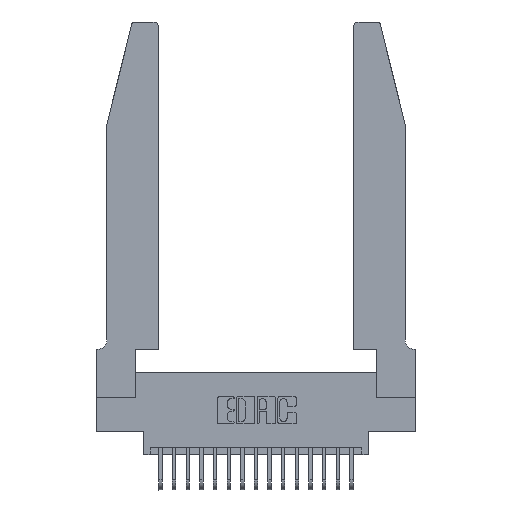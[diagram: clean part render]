
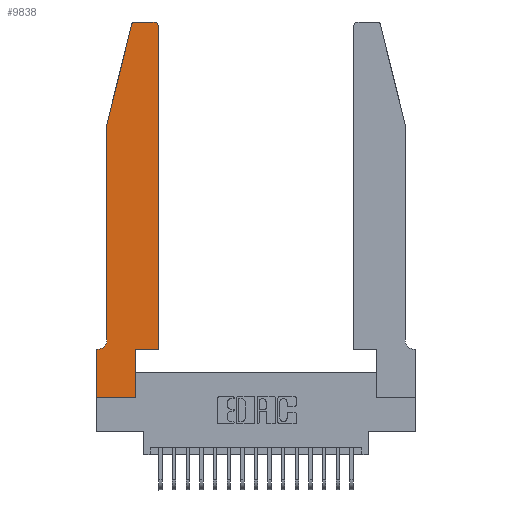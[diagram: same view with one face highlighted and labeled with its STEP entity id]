
A CAD part, top view. The second image highlights one B-rep face of the part: STEP entity #9838.
In plain terms, the highlighted planar face has unit normal (0, 0, 1).
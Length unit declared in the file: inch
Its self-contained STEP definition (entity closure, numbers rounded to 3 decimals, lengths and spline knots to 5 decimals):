
#3 = VERTEX_POINT ( 'NONE', #16463 ) ;
#255 = EDGE_CURVE ( 'NONE', #14930, #7111, #9008, .T. ) ;
#265 = CARTESIAN_POINT ( 'NONE',  ( 0.284, 2.75, 0.37 ) ) ;
#347 = CARTESIAN_POINT ( 'NONE',  ( 0.284, 2.72, 0.37 ) ) ;
#1038 = DIRECTION ( 'NONE',  ( 0., 0., 1. ) ) ;
#1170 = ORIENTED_EDGE ( 'NONE', *, *, #16123, .T. ) ;
#1214 = DIRECTION ( 'NONE',  ( 0., 1., 0. ) ) ;
#1330 = VECTOR ( 'NONE', #4417, 39.37008 ) ;
#1335 = DIRECTION ( 'NONE',  ( 1., 0., 0. ) ) ;
#1813 = VERTEX_POINT ( 'NONE', #8949 ) ;
#1991 = ORIENTED_EDGE ( 'NONE', *, *, #9637, .T. ) ;
#2097 = CARTESIAN_POINT ( 'NONE',  ( 0.4505, 2.72, 0.37 ) ) ;
#2104 = ORIENTED_EDGE ( 'NONE', *, *, #6098, .T. ) ;
#2173 = VECTOR ( 'NONE', #8226, 39.37008 ) ;
#2244 = EDGE_CURVE ( 'NONE', #2578, #7354, #13419, .T. ) ;
#2578 = VERTEX_POINT ( 'NONE', #265 ) ;
#2628 = EDGE_CURVE ( 'NONE', #7111, #5999, #11754, .T. ) ;
#2668 = LINE ( 'NONE', #11325, #2173 ) ;
#2983 = VECTOR ( 'NONE', #9840, 39.37008 ) ;
#3103 = AXIS2_PLACEMENT_3D ( 'NONE', #19707, #10705, #1335 ) ;
#3227 = CARTESIAN_POINT ( 'NONE',  ( 0.0755, 0.42, 0.37 ) ) ;
#3476 = DIRECTION ( 'NONE',  ( -1., 0., 0. ) ) ;
#3550 = AXIS2_PLACEMENT_3D ( 'NONE', #19565, #18955, #3476 ) ;
#3864 = VERTEX_POINT ( 'NONE', #2097 ) ;
#4045 = LINE ( 'NONE', #9313, #6709 ) ;
#4168 = CARTESIAN_POINT ( 'NONE',  ( 0.0755, 2., 0.37 ) ) ;
#4252 = ORIENTED_EDGE ( 'NONE', *, *, #18304, .T. ) ;
#4417 = DIRECTION ( 'NONE',  ( 0., -1., 0. ) ) ;
#4454 = ORIENTED_EDGE ( 'NONE', *, *, #9755, .T. ) ;
#4693 = DIRECTION ( 'NONE',  ( 1., 0., 0. ) ) ;
#4696 = ORIENTED_EDGE ( 'NONE', *, *, #11444, .T. ) ;
#4767 = ORIENTED_EDGE ( 'NONE', *, *, #12080, .T. ) ;
#4829 = DIRECTION ( 'NONE',  ( 0., 0., 1. ) ) ;
#4830 = ORIENTED_EDGE ( 'NONE', *, *, #18968, .T. ) ;
#4874 = CARTESIAN_POINT ( 'NONE',  ( 0.25487, 2.72718, 0.37 ) ) ;
#4988 = VERTEX_POINT ( 'NONE', #5011 ) ;
#5011 = CARTESIAN_POINT ( 'NONE',  ( 0.4505, 0.35, 0.37 ) ) ;
#5342 = AXIS2_PLACEMENT_3D ( 'NONE', #10432, #1038, #11948 ) ;
#5544 = LINE ( 'NONE', #7493, #1330 ) ;
#5623 = VECTOR ( 'NONE', #12862, 39.37008 ) ;
#5842 = VERTEX_POINT ( 'NONE', #12818 ) ;
#5999 = VERTEX_POINT ( 'NONE', #13427 ) ;
#6098 = EDGE_CURVE ( 'NONE', #3864, #3, #19409, .T. ) ;
#6588 = ORIENTED_EDGE ( 'NONE', *, *, #255, .T. ) ;
#6603 = DIRECTION ( 'NONE',  ( -0.239, -0.971, 0. ) ) ;
#6709 = VECTOR ( 'NONE', #19850, 39.37008 ) ;
#7096 = DIRECTION ( 'NONE',  ( 1., 0., 0. ) ) ;
#7111 = VERTEX_POINT ( 'NONE', #10537 ) ;
#7180 = DIRECTION ( 'NONE',  ( 0., -1., 0. ) ) ;
#7243 = LINE ( 'NONE', #16299, #19349 ) ;
#7354 = VERTEX_POINT ( 'NONE', #4874 ) ;
#7493 = CARTESIAN_POINT ( 'NONE',  ( 0.0755, 2., 0.37 ) ) ;
#8226 = DIRECTION ( 'NONE',  ( 1., 0., 0. ) ) ;
#8780 = VECTOR ( 'NONE', #7096, 39.37008 ) ;
#8949 = CARTESIAN_POINT ( 'NONE',  ( 0.2865, 0.35, 0.37 ) ) ;
#9008 = CIRCLE ( 'NONE', #3550, 0.07 ) ;
#9313 = CARTESIAN_POINT ( 'NONE',  ( 0.4505, 0.35, 0.37 ) ) ;
#9637 = EDGE_CURVE ( 'NONE', #3, #2578, #9763, .T. ) ;
#9755 = EDGE_CURVE ( 'NONE', #5842, #18118, #12348, .T. ) ;
#9763 = LINE ( 'NONE', #15817, #5623 ) ;
#9833 = VERTEX_POINT ( 'NONE', #4168 ) ;
#9838 = ADVANCED_FACE ( 'NONE', ( #18450 ), #19439, .T. ) ;
#9840 = DIRECTION ( 'NONE',  ( -1., 0., 0. ) ) ;
#10200 = ORIENTED_EDGE ( 'NONE', *, *, #2244, .T. ) ;
#10432 = CARTESIAN_POINT ( 'NONE',  ( 0., 0.35, 0.37 ) ) ;
#10537 = CARTESIAN_POINT ( 'NONE',  ( 0.0055, 0.35, 0.37 ) ) ;
#10705 = DIRECTION ( 'NONE',  ( 0., 0., 1. ) ) ;
#11325 = CARTESIAN_POINT ( 'NONE',  ( 0.4505, 0.35, 0.37 ) ) ;
#11336 = VECTOR ( 'NONE', #1214, 39.37008 ) ;
#11444 = EDGE_CURVE ( 'NONE', #9833, #14930, #5544, .T. ) ;
#11455 = ORIENTED_EDGE ( 'NONE', *, *, #2628, .T. ) ;
#11754 = LINE ( 'NONE', #18766, #2983 ) ;
#11948 = DIRECTION ( 'NONE',  ( 1., 0., 0. ) ) ;
#12080 = EDGE_CURVE ( 'NONE', #4988, #3864, #4045, .T. ) ;
#12348 = LINE ( 'NONE', #17714, #8780 ) ;
#12818 = CARTESIAN_POINT ( 'NONE',  ( 0., 0., 0.37 ) ) ;
#12862 = DIRECTION ( 'NONE',  ( -1., 0., 0. ) ) ;
#13419 = CIRCLE ( 'NONE', #17044, 0.03 ) ;
#13427 = CARTESIAN_POINT ( 'NONE',  ( 0., 0.35, 0.37 ) ) ;
#14337 = VECTOR ( 'NONE', #6603, 39.37008 ) ;
#14561 = EDGE_CURVE ( 'NONE', #7354, #9833, #18308, .T. ) ;
#14700 = CARTESIAN_POINT ( 'NONE',  ( 0.2865, 0., 0.37 ) ) ;
#14930 = VERTEX_POINT ( 'NONE', #3227 ) ;
#15332 = LINE ( 'NONE', #19601, #11336 ) ;
#15817 = CARTESIAN_POINT ( 'NONE',  ( 0.2605, 2.75, 0.37 ) ) ;
#16123 = EDGE_CURVE ( 'NONE', #1813, #4988, #2668, .T. ) ;
#16299 = CARTESIAN_POINT ( 'NONE',  ( 0., 0., 0.37 ) ) ;
#16463 = CARTESIAN_POINT ( 'NONE',  ( 0.4205, 2.75, 0.37 ) ) ;
#17044 = AXIS2_PLACEMENT_3D ( 'NONE', #347, #4829, #4693 ) ;
#17248 = CARTESIAN_POINT ( 'NONE',  ( 0.0755, 2., 0.37 ) ) ;
#17714 = CARTESIAN_POINT ( 'NONE',  ( 0., 0., 0.37 ) ) ;
#18118 = VERTEX_POINT ( 'NONE', #14700 ) ;
#18304 = EDGE_CURVE ( 'NONE', #18118, #1813, #15332, .T. ) ;
#18308 = LINE ( 'NONE', #17248, #14337 ) ;
#18450 = FACE_OUTER_BOUND ( 'NONE', #19364, .T. ) ;
#18766 = CARTESIAN_POINT ( 'NONE',  ( 0.0755, 0.35, 0.37 ) ) ;
#18955 = DIRECTION ( 'NONE',  ( 0., 0., -1. ) ) ;
#18968 = EDGE_CURVE ( 'NONE', #5999, #5842, #7243, .T. ) ;
#19337 = ORIENTED_EDGE ( 'NONE', *, *, #14561, .T. ) ;
#19349 = VECTOR ( 'NONE', #7180, 39.37008 ) ;
#19364 = EDGE_LOOP ( 'NONE', ( #1991, #10200, #19337, #4696, #6588, #11455, #4830, #4454, #4252, #1170, #4767, #2104 ) ) ;
#19409 = CIRCLE ( 'NONE', #3103, 0.03 ) ;
#19439 = PLANE ( 'NONE',  #5342 ) ;
#19565 = CARTESIAN_POINT ( 'NONE',  ( 0.0055, 0.42, 0.37 ) ) ;
#19601 = CARTESIAN_POINT ( 'NONE',  ( 0.2865, 0.35, 0.37 ) ) ;
#19707 = CARTESIAN_POINT ( 'NONE',  ( 0.4205, 2.72, 0.37 ) ) ;
#19850 = DIRECTION ( 'NONE',  ( 0., 1., 0. ) ) ;
